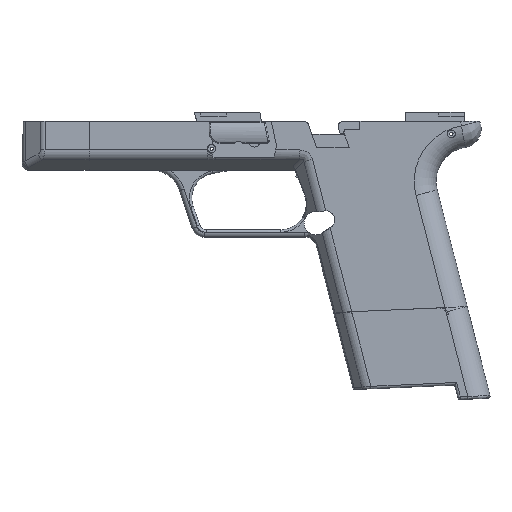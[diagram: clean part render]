
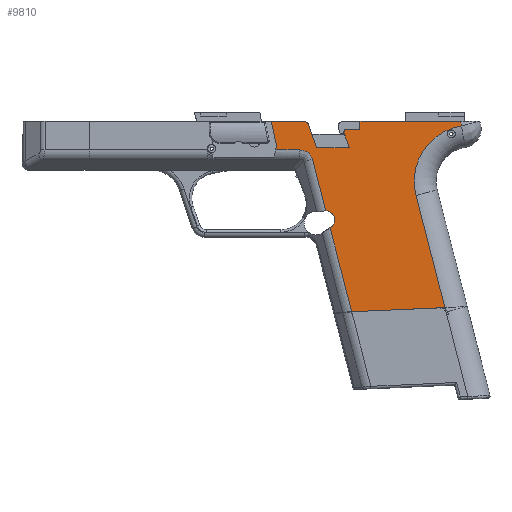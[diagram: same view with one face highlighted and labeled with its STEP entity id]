
A CAD part, left-side view. The second image highlights one B-rep face of the part: STEP entity #9810.
In plain terms, the highlighted face is planar.
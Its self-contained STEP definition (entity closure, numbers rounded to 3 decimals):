
#110=ELLIPSE('',#10613,10.693,7.);
#630=PLANE('',#10611);
#1015=FACE_OUTER_BOUND('',#1583,.T.);
#1583=EDGE_LOOP('',(#7687,#7688,#7689,#7690,#7691,#7692,#7693,#7694,#7695,
#7696,#7697,#7698,#7699,#7700,#7701,#7702,#7703,#7704,#7705,#7706,#7707,
#7708,#7709));
#2322=LINE('',#16121,#3242);
#2323=LINE('',#16123,#3243);
#2324=LINE('',#16125,#3244);
#2325=LINE('',#16129,#3245);
#2326=LINE('',#16131,#3246);
#2327=LINE('',#16133,#3247);
#2328=LINE('',#16135,#3248);
#2329=LINE('',#16139,#3249);
#2330=LINE('',#16147,#3250);
#2331=LINE('',#16149,#3251);
#2332=LINE('',#16151,#3252);
#2333=LINE('',#16153,#3253);
#2334=LINE('',#16159,#3254);
#2335=LINE('',#16161,#3255);
#2336=LINE('',#16162,#3256);
#3242=VECTOR('',#12367,10.);
#3243=VECTOR('',#12368,10.);
#3244=VECTOR('',#12369,10.);
#3245=VECTOR('',#12372,10.);
#3246=VECTOR('',#12373,10.);
#3247=VECTOR('',#12374,10.);
#3248=VECTOR('',#12375,10.);
#3249=VECTOR('',#12378,10.);
#3250=VECTOR('',#12385,10.);
#3251=VECTOR('',#12386,10.);
#3252=VECTOR('',#12387,10.);
#3253=VECTOR('',#12388,10.);
#3254=VECTOR('',#12393,10.);
#3255=VECTOR('',#12394,10.);
#3256=VECTOR('',#12395,10.);
#3876=CIRCLE('',#10610,1.);
#3877=CIRCLE('',#10612,2.);
#3878=CIRCLE('',#10614,3.585);
#3879=CIRCLE('',#10615,2.921);
#3880=CIRCLE('',#10616,3.585);
#3881=CIRCLE('',#10617,22.475);
#3882=CIRCLE('',#10618,7.5);
#4446=VERTEX_POINT('',#16114);
#4447=VERTEX_POINT('',#16116);
#4448=VERTEX_POINT('',#16120);
#4449=VERTEX_POINT('',#16122);
#4450=VERTEX_POINT('',#16124);
#4451=VERTEX_POINT('',#16126);
#4452=VERTEX_POINT('',#16128);
#4453=VERTEX_POINT('',#16130);
#4454=VERTEX_POINT('',#16132);
#4455=VERTEX_POINT('',#16134);
#4456=VERTEX_POINT('',#16136);
#4457=VERTEX_POINT('',#16138);
#4458=VERTEX_POINT('',#16140);
#4459=VERTEX_POINT('',#16142);
#4460=VERTEX_POINT('',#16144);
#4461=VERTEX_POINT('',#16146);
#4462=VERTEX_POINT('',#16148);
#4463=VERTEX_POINT('',#16150);
#4464=VERTEX_POINT('',#16152);
#4465=VERTEX_POINT('',#16154);
#4466=VERTEX_POINT('',#16156);
#4467=VERTEX_POINT('',#16158);
#4468=VERTEX_POINT('',#16160);
#5608=EDGE_CURVE('',#4446,#4447,#3876,.T.);
#5610=EDGE_CURVE('',#4446,#4448,#2322,.F.);
#5611=EDGE_CURVE('',#4448,#4449,#2323,.T.);
#5612=EDGE_CURVE('',#4449,#4450,#2324,.F.);
#5613=EDGE_CURVE('',#4451,#4450,#3877,.T.);
#5614=EDGE_CURVE('',#4451,#4452,#2325,.T.);
#5615=EDGE_CURVE('',#4452,#4453,#2326,.T.);
#5616=EDGE_CURVE('',#4453,#4454,#2327,.T.);
#5617=EDGE_CURVE('',#4455,#4454,#2328,.T.);
#5618=EDGE_CURVE('',#4456,#4455,#110,.T.);
#5619=EDGE_CURVE('',#4457,#4456,#2329,.T.);
#5620=EDGE_CURVE('',#4457,#4458,#3878,.T.);
#5621=EDGE_CURVE('',#4458,#4459,#3879,.T.);
#5622=EDGE_CURVE('',#4459,#4460,#3880,.T.);
#5623=EDGE_CURVE('',#4460,#4461,#2330,.T.);
#5624=EDGE_CURVE('',#4462,#4461,#2331,.T.);
#5625=EDGE_CURVE('',#4463,#4462,#2332,.T.);
#5626=EDGE_CURVE('',#4464,#4463,#2333,.T.);
#5627=EDGE_CURVE('',#4465,#4464,#3881,.T.);
#5628=EDGE_CURVE('',#4466,#4465,#3882,.T.);
#5629=EDGE_CURVE('',#4466,#4467,#2334,.T.);
#5630=EDGE_CURVE('',#4467,#4468,#2335,.F.);
#5631=EDGE_CURVE('',#4468,#4447,#2336,.T.);
#7687=ORIENTED_EDGE('',*,*,#5608,.F.);
#7688=ORIENTED_EDGE('',*,*,#5610,.T.);
#7689=ORIENTED_EDGE('',*,*,#5611,.T.);
#7690=ORIENTED_EDGE('',*,*,#5612,.T.);
#7691=ORIENTED_EDGE('',*,*,#5613,.F.);
#7692=ORIENTED_EDGE('',*,*,#5614,.T.);
#7693=ORIENTED_EDGE('',*,*,#5615,.T.);
#7694=ORIENTED_EDGE('',*,*,#5616,.T.);
#7695=ORIENTED_EDGE('',*,*,#5617,.F.);
#7696=ORIENTED_EDGE('',*,*,#5618,.F.);
#7697=ORIENTED_EDGE('',*,*,#5619,.F.);
#7698=ORIENTED_EDGE('',*,*,#5620,.T.);
#7699=ORIENTED_EDGE('',*,*,#5621,.T.);
#7700=ORIENTED_EDGE('',*,*,#5622,.T.);
#7701=ORIENTED_EDGE('',*,*,#5623,.T.);
#7702=ORIENTED_EDGE('',*,*,#5624,.F.);
#7703=ORIENTED_EDGE('',*,*,#5625,.F.);
#7704=ORIENTED_EDGE('',*,*,#5626,.F.);
#7705=ORIENTED_EDGE('',*,*,#5627,.F.);
#7706=ORIENTED_EDGE('',*,*,#5628,.F.);
#7707=ORIENTED_EDGE('',*,*,#5629,.T.);
#7708=ORIENTED_EDGE('',*,*,#5630,.T.);
#7709=ORIENTED_EDGE('',*,*,#5631,.T.);
#9810=ADVANCED_FACE('',(#1015),#630,.F.);
#10610=AXIS2_PLACEMENT_3D('',#16117,#12362,#12363);
#10611=AXIS2_PLACEMENT_3D('',#16119,#12365,#12366);
#10612=AXIS2_PLACEMENT_3D('',#16127,#12370,#12371);
#10613=AXIS2_PLACEMENT_3D('',#16137,#12376,#12377);
#10614=AXIS2_PLACEMENT_3D('',#16141,#12379,#12380);
#10615=AXIS2_PLACEMENT_3D('',#16143,#12381,#12382);
#10616=AXIS2_PLACEMENT_3D('',#16145,#12383,#12384);
#10617=AXIS2_PLACEMENT_3D('',#16155,#12389,#12390);
#10618=AXIS2_PLACEMENT_3D('',#16157,#12391,#12392);
#12362=DIRECTION('center_axis',(-1.,0.,0.));
#12363=DIRECTION('ref_axis',(0.,0.817,-0.576));
#12365=DIRECTION('center_axis',(-1.,0.,0.));
#12366=DIRECTION('ref_axis',(0.,1.,0.));
#12367=DIRECTION('',(0.,0.336,-0.942));
#12368=DIRECTION('',(0.,1.,0.));
#12369=DIRECTION('',(0.,-0.336,0.942));
#12370=DIRECTION('center_axis',(-1.,0.,0.));
#12371=DIRECTION('ref_axis',(0.,-0.576,-0.817));
#12372=DIRECTION('',(0.,1.,0.));
#12373=DIRECTION('',(0.,-0.21,0.978));
#12374=DIRECTION('',(0.,0.21,0.978));
#12375=DIRECTION('',(0.,1.,0.));
#12376=DIRECTION('center_axis',(1.,0.,0.));
#12377=DIRECTION('ref_axis',(0.,-0.714,-0.7));
#12378=DIRECTION('',(0.,0.249,-0.969));
#12379=DIRECTION('center_axis',(-1.,0.,0.));
#12380=DIRECTION('ref_axis',(0.,1.,0.));
#12381=DIRECTION('center_axis',(-1.,0.,0.));
#12382=DIRECTION('ref_axis',(0.,1.,0.));
#12383=DIRECTION('center_axis',(-1.,0.,0.));
#12384=DIRECTION('ref_axis',(0.,1.,0.));
#12385=DIRECTION('',(0.,0.828,0.56));
#12386=DIRECTION('',(0.,0.249,-0.969));
#12387=DIRECTION('',(0.,0.999,0.044));
#12388=DIRECTION('',(0.,-0.249,0.969));
#12389=DIRECTION('center_axis',(1.,0.,0.));
#12390=DIRECTION('ref_axis',(0.,0.,1.));
#12391=DIRECTION('center_axis',(1.,0.,0.));
#12392=DIRECTION('ref_axis',(0.,-0.97,-0.244));
#12393=DIRECTION('',(0.,1.,0.));
#12394=DIRECTION('',(0.,0.,-1.));
#12395=DIRECTION('',(0.,1.,0.));
#16114=CARTESIAN_POINT('',(22.175,-34.374,-2.995));
#16116=CARTESIAN_POINT('',(22.175,-35.316,-4.331));
#16117=CARTESIAN_POINT('Origin',(22.175,-35.316,-3.331));
#16119=CARTESIAN_POINT('Origin',(22.175,-7.921,2.186));
#16120=CARTESIAN_POINT('',(22.175,-36.514,3.));
#16121=CARTESIAN_POINT('',(22.175,-32.976,-6.913));
#16122=CARTESIAN_POINT('',(22.175,-23.407,3.));
#16123=CARTESIAN_POINT('',(22.175,-23.764,3.));
#16124=CARTESIAN_POINT('',(22.175,-20.114,-6.228));
#16125=CARTESIAN_POINT('',(22.175,-21.552,-2.199));
#16126=CARTESIAN_POINT('',(22.175,-18.23,-7.556));
#16127=CARTESIAN_POINT('Origin',(22.175,-18.23,-5.556));
#16128=CARTESIAN_POINT('',(22.175,-5.3,-7.556));
#16129=CARTESIAN_POINT('',(22.175,-86.951,-7.556));
#16130=CARTESIAN_POINT('',(22.175,-7.389,2.186));
#16131=CARTESIAN_POINT('',(22.175,-6.356,-2.63));
#16132=CARTESIAN_POINT('',(22.175,-7.025,3.884));
#16133=CARTESIAN_POINT('',(22.175,-7.4,2.132));
#16134=CARTESIAN_POINT('',(22.175,-16.536,3.884));
#16135=CARTESIAN_POINT('',(22.175,33.814,3.884));
#16136=CARTESIAN_POINT('',(22.175,-21.783,7.651));
#16137=CARTESIAN_POINT('Origin',(22.175,-12.907,12.884));
#16138=CARTESIAN_POINT('',(22.175,-27.074,28.233));
#16139=CARTESIAN_POINT('',(22.175,-26.659,26.619));
#16140=CARTESIAN_POINT('',(22.175,-30.502,30.561));
#16141=CARTESIAN_POINT('Origin',(22.175,-27.144,31.817));
#16142=CARTESIAN_POINT('',(22.175,-30.617,30.925));
#16143=CARTESIAN_POINT('Origin',(22.175,-27.779,31.618));
#16144=CARTESIAN_POINT('',(22.175,-29.153,34.787));
#16145=CARTESIAN_POINT('Origin',(22.175,-27.144,31.817));
#16146=CARTESIAN_POINT('',(22.175,-28.817,35.014));
#16147=CARTESIAN_POINT('',(22.175,-27.054,36.207));
#16148=CARTESIAN_POINT('',(22.175,-37.447,68.587));
#16149=CARTESIAN_POINT('',(22.175,-26.659,26.619));
#16150=CARTESIAN_POINT('',(22.175,-74.722,66.935));
#16151=CARTESIAN_POINT('',(22.175,-40.785,68.439));
#16152=CARTESIAN_POINT('',(22.175,-63.184,22.049));
#16153=CARTESIAN_POINT('',(22.175,-75.103,68.418));
#16154=CARTESIAN_POINT('',(22.175,-81.332,-5.728));
#16155=CARTESIAN_POINT('Origin',(22.175,-84.951,16.453));
#16156=CARTESIAN_POINT('',(22.175,-81.106,-7.556));
#16157=CARTESIAN_POINT('Origin',(22.175,-88.606,-7.556));
#16158=CARTESIAN_POINT('',(22.175,-40.774,-7.556));
#16159=CARTESIAN_POINT('',(22.175,-84.951,-7.556));
#16160=CARTESIAN_POINT('',(22.175,-40.774,-4.331));
#16161=CARTESIAN_POINT('',(22.175,-40.774,-2.685));
#16162=CARTESIAN_POINT('',(22.175,-20.598,-4.331));
